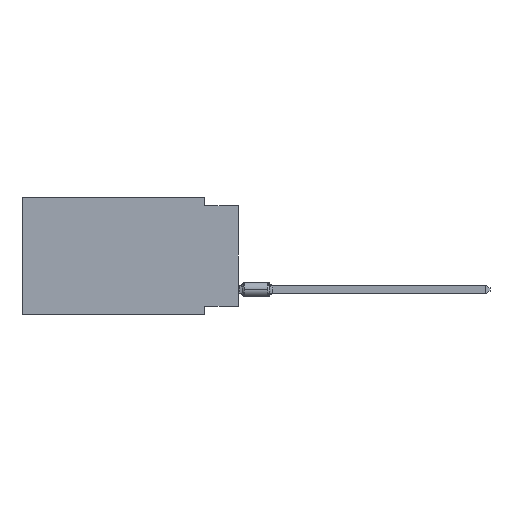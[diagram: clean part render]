
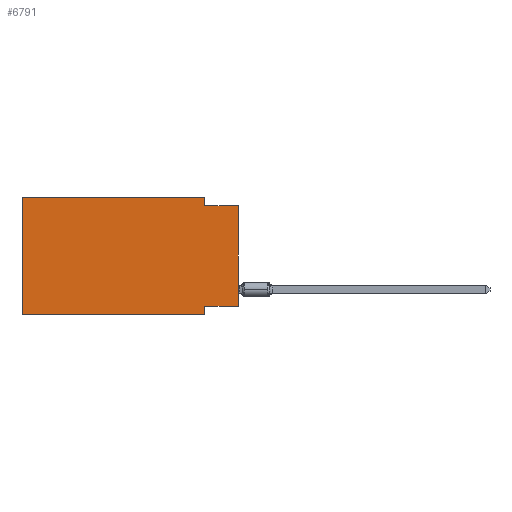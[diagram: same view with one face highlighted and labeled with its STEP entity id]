
A CAD part, left-side view. The second image highlights one B-rep face of the part: STEP entity #6791.
In plain terms, the highlighted planar face has unit normal (-1, 0, 0).
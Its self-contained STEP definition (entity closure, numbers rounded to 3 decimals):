
#706 = EDGE_LOOP ( 'NONE', ( #21144, #20447, #15888, #11172, #13762, #14437, #8857, #17483 ) ) ;
#1661 = EDGE_CURVE ( 'NONE', #12047, #13296, #11899, .T. ) ;
#1809 = DIRECTION ( 'NONE',  ( 0., -1., 0. ) ) ;
#2001 = DIRECTION ( 'NONE',  ( 0., 0., -1. ) ) ;
#2345 = VERTEX_POINT ( 'NONE', #15164 ) ;
#2370 = CARTESIAN_POINT ( 'NONE',  ( 0., 0., -8.255 ) ) ;
#3074 = DIRECTION ( 'NONE',  ( 0., 1., 0. ) ) ;
#3189 = FACE_OUTER_BOUND ( 'NONE', #706, .T. ) ;
#3509 = DIRECTION ( 'NONE',  ( 1., 0., 0. ) ) ;
#3657 = VECTOR ( 'NONE', #1809, 1000. ) ;
#3954 = LINE ( 'NONE', #10971, #5290 ) ;
#4448 = DIRECTION ( 'NONE',  ( 0., 0., -1. ) ) ;
#4603 = DIRECTION ( 'NONE',  ( 0., 0., 1. ) ) ;
#4791 = CARTESIAN_POINT ( 'NONE',  ( 0., 2.54, -8.89 ) ) ;
#4876 = CARTESIAN_POINT ( 'NONE',  ( 0., 0., -8.255 ) ) ;
#5030 = VECTOR ( 'NONE', #4448, 1000. ) ;
#5290 = VECTOR ( 'NONE', #21289, 1000. ) ;
#5471 = CARTESIAN_POINT ( 'NONE',  ( 0., 0., -0.635 ) ) ;
#5602 = LINE ( 'NONE', #13985, #6237 ) ;
#6237 = VECTOR ( 'NONE', #12295, 1000. ) ;
#6260 = CARTESIAN_POINT ( 'NONE',  ( 0., 16.383, 0. ) ) ;
#6791 = ADVANCED_FACE ( 'NONE', ( #3189 ), #13818, .F. ) ;
#6804 = DIRECTION ( 'NONE',  ( 0., 0., -1. ) ) ;
#6807 = CARTESIAN_POINT ( 'NONE',  ( 0., 16.383, 0. ) ) ;
#6887 = CARTESIAN_POINT ( 'NONE',  ( 0., 2.54, 0. ) ) ;
#7539 = CARTESIAN_POINT ( 'NONE',  ( 0., 16.383, -8.89 ) ) ;
#8697 = VERTEX_POINT ( 'NONE', #18317 ) ;
#8719 = EDGE_CURVE ( 'NONE', #12047, #20575, #20026, .T. ) ;
#8857 = ORIENTED_EDGE ( 'NONE', *, *, #20651, .F. ) ;
#9608 = EDGE_CURVE ( 'NONE', #10159, #2345, #10388, .T. ) ;
#9689 = CARTESIAN_POINT ( 'NONE',  ( 0., 0., 0. ) ) ;
#10159 = VERTEX_POINT ( 'NONE', #12800 ) ;
#10365 = VECTOR ( 'NONE', #12023, 1000. ) ;
#10388 = LINE ( 'NONE', #6887, #18650 ) ;
#10531 = AXIS2_PLACEMENT_3D ( 'NONE', #11796, #3509, #6804 ) ;
#10971 = CARTESIAN_POINT ( 'NONE',  ( 0., 16.383, 0. ) ) ;
#11172 = ORIENTED_EDGE ( 'NONE', *, *, #13909, .F. ) ;
#11580 = CARTESIAN_POINT ( 'NONE',  ( 0., 0., -0.635 ) ) ;
#11796 = CARTESIAN_POINT ( 'NONE',  ( 0., 16.383, 0. ) ) ;
#11899 = LINE ( 'NONE', #4876, #18797 ) ;
#12023 = DIRECTION ( 'NONE',  ( 0., -1., 0. ) ) ;
#12047 = VERTEX_POINT ( 'NONE', #2370 ) ;
#12295 = DIRECTION ( 'NONE',  ( 0., -1., 0. ) ) ;
#12800 = CARTESIAN_POINT ( 'NONE',  ( 0., 2.54, 0. ) ) ;
#13119 = CARTESIAN_POINT ( 'NONE',  ( 0., 2.54, -8.255 ) ) ;
#13296 = VERTEX_POINT ( 'NONE', #13119 ) ;
#13605 = EDGE_CURVE ( 'NONE', #15599, #8697, #5602, .T. ) ;
#13762 = ORIENTED_EDGE ( 'NONE', *, *, #17022, .F. ) ;
#13818 = PLANE ( 'NONE',  #10531 ) ;
#13909 = EDGE_CURVE ( 'NONE', #21844, #10159, #22339, .T. ) ;
#13985 = CARTESIAN_POINT ( 'NONE',  ( 0., 16.383, -8.89 ) ) ;
#14437 = ORIENTED_EDGE ( 'NONE', *, *, #13605, .T. ) ;
#15164 = CARTESIAN_POINT ( 'NONE',  ( 0., 2.54, -0.635 ) ) ;
#15599 = VERTEX_POINT ( 'NONE', #7539 ) ;
#15888 = ORIENTED_EDGE ( 'NONE', *, *, #9608, .F. ) ;
#16161 = VECTOR ( 'NONE', #4603, 1000. ) ;
#16700 = EDGE_CURVE ( 'NONE', #2345, #20575, #16912, .T. ) ;
#16801 = LINE ( 'NONE', #4791, #5030 ) ;
#16912 = LINE ( 'NONE', #11580, #10365 ) ;
#17022 = EDGE_CURVE ( 'NONE', #15599, #21844, #3954, .T. ) ;
#17483 = ORIENTED_EDGE ( 'NONE', *, *, #1661, .F. ) ;
#18317 = CARTESIAN_POINT ( 'NONE',  ( 0., 2.54, -8.89 ) ) ;
#18650 = VECTOR ( 'NONE', #2001, 1000. ) ;
#18797 = VECTOR ( 'NONE', #3074, 1000. ) ;
#20026 = LINE ( 'NONE', #9689, #16161 ) ;
#20447 = ORIENTED_EDGE ( 'NONE', *, *, #16700, .F. ) ;
#20575 = VERTEX_POINT ( 'NONE', #5471 ) ;
#20651 = EDGE_CURVE ( 'NONE', #13296, #8697, #16801, .T. ) ;
#21144 = ORIENTED_EDGE ( 'NONE', *, *, #8719, .T. ) ;
#21289 = DIRECTION ( 'NONE',  ( 0., 0., 1. ) ) ;
#21844 = VERTEX_POINT ( 'NONE', #6260 ) ;
#22339 = LINE ( 'NONE', #6807, #3657 ) ;
